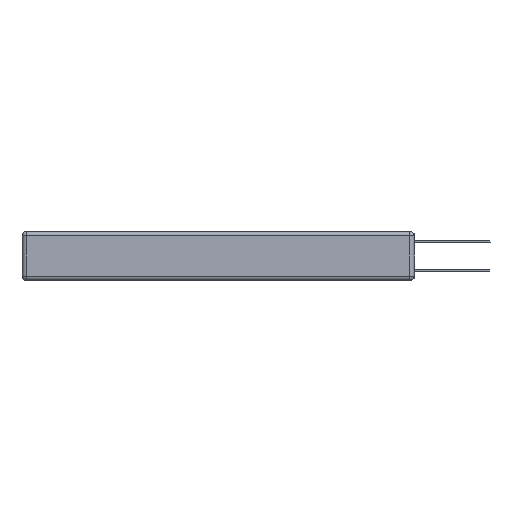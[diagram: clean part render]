
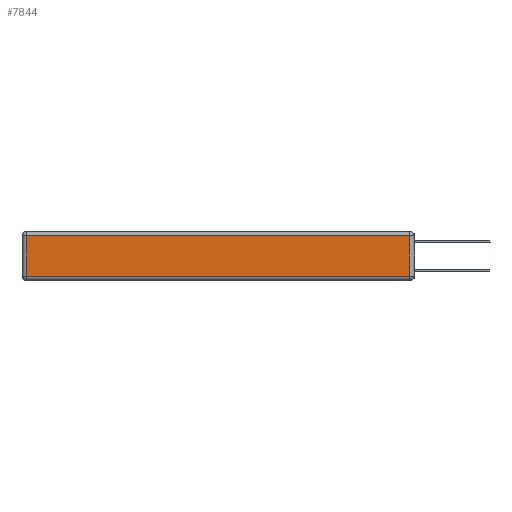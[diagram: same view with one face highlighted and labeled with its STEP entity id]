
A CAD part, left-side view. The second image highlights one B-rep face of the part: STEP entity #7844.
In plain terms, the highlighted planar face has unit normal (-1, 0, 0).
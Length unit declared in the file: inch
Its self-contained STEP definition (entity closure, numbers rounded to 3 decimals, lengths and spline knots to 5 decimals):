
#109 = VECTOR ( 'NONE', #1371, 39.37008 ) ;
#848 = VERTEX_POINT ( 'NONE', #4863 ) ;
#1371 = DIRECTION ( 'NONE',  ( 0., 0., 1. ) ) ;
#1522 = EDGE_CURVE ( 'NONE', #6928, #15062, #5851, .T. ) ;
#2120 = DIRECTION ( 'NONE',  ( 0., 0., 1. ) ) ;
#2383 = EDGE_CURVE ( 'NONE', #18327, #848, #11010, .T. ) ;
#2502 = DIRECTION ( 'NONE',  ( 0., 1., 0. ) ) ;
#2577 = DIRECTION ( 'NONE',  ( 0., 0., -1. ) ) ;
#2860 = LINE ( 'NONE', #3635, #7369 ) ;
#3496 = EDGE_CURVE ( 'NONE', #15062, #18327, #18121, .T. ) ;
#3635 = CARTESIAN_POINT ( 'NONE',  ( 0., 2.72, -0.343 ) ) ;
#4863 = CARTESIAN_POINT ( 'NONE',  ( 0., 2.72, -0.03 ) ) ;
#4895 = VECTOR ( 'NONE', #2502, 39.37008 ) ;
#5851 = LINE ( 'NONE', #13839, #8358 ) ;
#6541 = DIRECTION ( 'NONE',  ( -1., 0., 0. ) ) ;
#6687 = DIRECTION ( 'NONE',  ( 0., -1., 0. ) ) ;
#6721 = FACE_OUTER_BOUND ( 'NONE', #9459, .T. ) ;
#6928 = VERTEX_POINT ( 'NONE', #9389 ) ;
#7369 = VECTOR ( 'NONE', #2577, 39.37008 ) ;
#7375 = ORIENTED_EDGE ( 'NONE', *, *, #9514, .T. ) ;
#7783 = CARTESIAN_POINT ( 'NONE',  ( 0., 0.03, -0.03 ) ) ;
#7844 = ADVANCED_FACE ( 'NONE', ( #6721 ), #13545, .T. ) ;
#8358 = VECTOR ( 'NONE', #6687, 39.37008 ) ;
#8537 = ORIENTED_EDGE ( 'NONE', *, *, #2383, .T. ) ;
#9389 = CARTESIAN_POINT ( 'NONE',  ( 0., 2.72, -0.313 ) ) ;
#9459 = EDGE_LOOP ( 'NONE', ( #10099, #15793, #8537, #7375 ) ) ;
#9514 = EDGE_CURVE ( 'NONE', #848, #6928, #2860, .T. ) ;
#10012 = CARTESIAN_POINT ( 'NONE',  ( 0., 0.03, -0.343 ) ) ;
#10099 = ORIENTED_EDGE ( 'NONE', *, *, #1522, .T. ) ;
#11010 = LINE ( 'NONE', #14146, #4895 ) ;
#13345 = AXIS2_PLACEMENT_3D ( 'NONE', #15008, #6541, #2120 ) ;
#13545 = PLANE ( 'NONE',  #13345 ) ;
#13839 = CARTESIAN_POINT ( 'NONE',  ( 0., 0., -0.313 ) ) ;
#13930 = CARTESIAN_POINT ( 'NONE',  ( 0., 0.03, -0.313 ) ) ;
#14146 = CARTESIAN_POINT ( 'NONE',  ( 0., 2.75, -0.03 ) ) ;
#15008 = CARTESIAN_POINT ( 'NONE',  ( 0., 0., -0.343 ) ) ;
#15062 = VERTEX_POINT ( 'NONE', #13930 ) ;
#15793 = ORIENTED_EDGE ( 'NONE', *, *, #3496, .T. ) ;
#18121 = LINE ( 'NONE', #10012, #109 ) ;
#18327 = VERTEX_POINT ( 'NONE', #7783 ) ;
